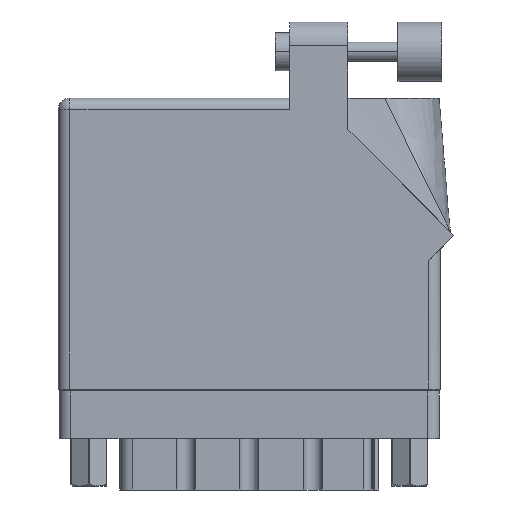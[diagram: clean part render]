
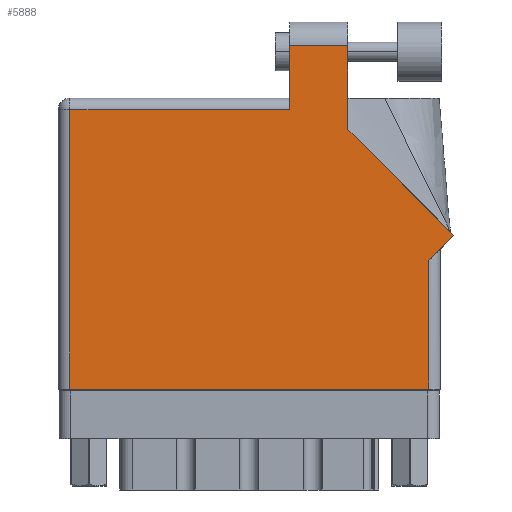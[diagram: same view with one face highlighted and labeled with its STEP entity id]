
A CAD part, front view. The second image highlights one B-rep face of the part: STEP entity #5888.
In plain terms, the highlighted face is planar.
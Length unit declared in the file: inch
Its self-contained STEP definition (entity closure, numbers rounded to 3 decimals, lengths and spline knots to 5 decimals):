
#252 = CARTESIAN_POINT ( 'NONE',  ( 0., 1.468, 0. ) ) ;
#821 = CARTESIAN_POINT ( 'NONE',  ( 2.08071, 0.80771, 0. ) ) ;
#1709 = VERTEX_POINT ( 'NONE', #17569 ) ;
#3363 = EDGE_CURVE ( 'NONE', #47466, #16039, #39183, .T. ) ;
#5348 = VERTEX_POINT ( 'NONE', #27046 ) ;
#5440 = DIRECTION ( 'NONE',  ( 0., 1., 0. ) ) ;
#5888 = ADVANCED_FACE ( 'NONE', ( #28705 ), #30397, .F. ) ;
#6032 = DIRECTION ( 'NONE',  ( 0., -1., 0. ) ) ;
#6679 = CARTESIAN_POINT ( 'NONE',  ( 1.948, 0.675, 0. ) ) ;
#7013 = CARTESIAN_POINT ( 'NONE',  ( 0., 1.53, 0. ) ) ;
#7616 = EDGE_CURVE ( 'NONE', #16039, #1709, #19532, .T. ) ;
#7853 = VECTOR ( 'NONE', #21597, 39.37008 ) ;
#7918 = VECTOR ( 'NONE', #46925, 39.37008 ) ;
#9467 = LINE ( 'NONE', #25246, #49273 ) ;
#9837 = EDGE_LOOP ( 'NONE', ( #15188, #35654, #45668, #38974, #45396, #38646, #25031, #31500, #14444 ) ) ;
#10281 = LINE ( 'NONE', #29516, #7853 ) ;
#10578 = VERTEX_POINT ( 'NONE', #48193 ) ;
#10665 = DIRECTION ( 'NONE',  ( 0., -1., 0. ) ) ;
#10740 = EDGE_CURVE ( 'NONE', #33836, #12628, #32428, .T. ) ;
#11238 = DIRECTION ( 'NONE',  ( -1., 0., 0. ) ) ;
#11385 = CARTESIAN_POINT ( 'NONE',  ( 2.01, 0.737, 0. ) ) ;
#12628 = VERTEX_POINT ( 'NONE', #23987 ) ;
#13082 = VERTEX_POINT ( 'NONE', #30559 ) ;
#14444 = ORIENTED_EDGE ( 'NONE', *, *, #26737, .T. ) ;
#15188 = ORIENTED_EDGE ( 'NONE', *, *, #36105, .T. ) ;
#16039 = VERTEX_POINT ( 'NONE', #39555 ) ;
#16676 = DIRECTION ( 'NONE',  ( -1., 0., 0. ) ) ;
#17569 = CARTESIAN_POINT ( 'NONE',  ( 0.062, 1.468, 0. ) ) ;
#18179 = VECTOR ( 'NONE', #30466, 39.37008 ) ;
#18273 = AXIS2_PLACEMENT_3D ( 'NONE', #7013, #26336, #11238 ) ;
#19054 = LINE ( 'NONE', #32368, #28710 ) ;
#19532 = LINE ( 'NONE', #252, #38859 ) ;
#21597 = DIRECTION ( 'NONE',  ( 1., 0., 0. ) ) ;
#23384 = VECTOR ( 'NONE', #6032, 39.37008 ) ;
#23987 = CARTESIAN_POINT ( 'NONE',  ( 2.08071, 0.80771, 0. ) ) ;
#24220 = LINE ( 'NONE', #26077, #18179 ) ;
#24890 = VERTEX_POINT ( 'NONE', #39587 ) ;
#25031 = ORIENTED_EDGE ( 'NONE', *, *, #39712, .T. ) ;
#25246 = CARTESIAN_POINT ( 'NONE',  ( 1.524, 1.36442, 0. ) ) ;
#26077 = CARTESIAN_POINT ( 'NONE',  ( 1.948, 0.737, 0. ) ) ;
#26336 = DIRECTION ( 'NONE',  ( 0., 0., -1. ) ) ;
#26737 = EDGE_CURVE ( 'NONE', #12628, #10578, #28345, .T. ) ;
#27046 = CARTESIAN_POINT ( 'NONE',  ( 1.524, 1.805, 0. ) ) ;
#28345 = LINE ( 'NONE', #821, #7918 ) ;
#28705 = FACE_OUTER_BOUND ( 'NONE', #9837, .T. ) ;
#28710 = VECTOR ( 'NONE', #29136, 39.37008 ) ;
#28882 = VECTOR ( 'NONE', #10665, 39.37008 ) ;
#29136 = DIRECTION ( 'NONE',  ( -1., 0., 0. ) ) ;
#29516 = CARTESIAN_POINT ( 'NONE',  ( 0., 0., 0. ) ) ;
#30397 = PLANE ( 'NONE',  #18273 ) ;
#30466 = DIRECTION ( 'NONE',  ( 0., 1., 0. ) ) ;
#30559 = CARTESIAN_POINT ( 'NONE',  ( 1.948, 0., 0. ) ) ;
#31500 = ORIENTED_EDGE ( 'NONE', *, *, #10740, .T. ) ;
#31857 = VECTOR ( 'NONE', #34607, 39.37008 ) ;
#32368 = CARTESIAN_POINT ( 'NONE',  ( 1.217, 1.805, 0. ) ) ;
#32428 = LINE ( 'NONE', #11385, #31857 ) ;
#33660 = LINE ( 'NONE', #45078, #23384 ) ;
#33836 = VERTEX_POINT ( 'NONE', #6679 ) ;
#34607 = DIRECTION ( 'NONE',  ( 0.707, 0.707, 0. ) ) ;
#34872 = EDGE_CURVE ( 'NONE', #1709, #24890, #33660, .T. ) ;
#35654 = ORIENTED_EDGE ( 'NONE', *, *, #36121, .T. ) ;
#36105 = EDGE_CURVE ( 'NONE', #10578, #5348, #9467, .T. ) ;
#36121 = EDGE_CURVE ( 'NONE', #5348, #47466, #19054, .T. ) ;
#38646 = ORIENTED_EDGE ( 'NONE', *, *, #41432, .T. ) ;
#38859 = VECTOR ( 'NONE', #16676, 39.37008 ) ;
#38974 = ORIENTED_EDGE ( 'NONE', *, *, #7616, .T. ) ;
#39183 = LINE ( 'NONE', #41966, #28882 ) ;
#39555 = CARTESIAN_POINT ( 'NONE',  ( 1.217, 1.468, 0. ) ) ;
#39587 = CARTESIAN_POINT ( 'NONE',  ( 0.062, 0., 0. ) ) ;
#39712 = EDGE_CURVE ( 'NONE', #13082, #33836, #24220, .T. ) ;
#41432 = EDGE_CURVE ( 'NONE', #24890, #13082, #10281, .T. ) ;
#41966 = CARTESIAN_POINT ( 'NONE',  ( 1.217, 1.53, 0. ) ) ;
#44905 = CARTESIAN_POINT ( 'NONE',  ( 1.217, 1.805, 0. ) ) ;
#45078 = CARTESIAN_POINT ( 'NONE',  ( 0.062, 0., 0. ) ) ;
#45396 = ORIENTED_EDGE ( 'NONE', *, *, #34872, .T. ) ;
#45668 = ORIENTED_EDGE ( 'NONE', *, *, #3363, .T. ) ;
#46925 = DIRECTION ( 'NONE',  ( -0.707, 0.707, 0. ) ) ;
#47466 = VERTEX_POINT ( 'NONE', #44905 ) ;
#48193 = CARTESIAN_POINT ( 'NONE',  ( 1.524, 1.36442, 0. ) ) ;
#49273 = VECTOR ( 'NONE', #5440, 39.37008 ) ;
